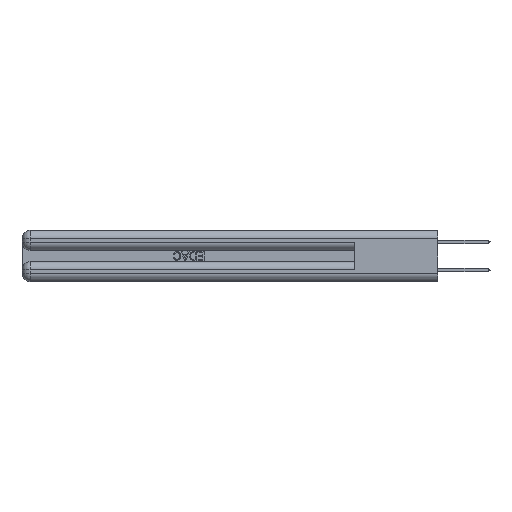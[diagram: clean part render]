
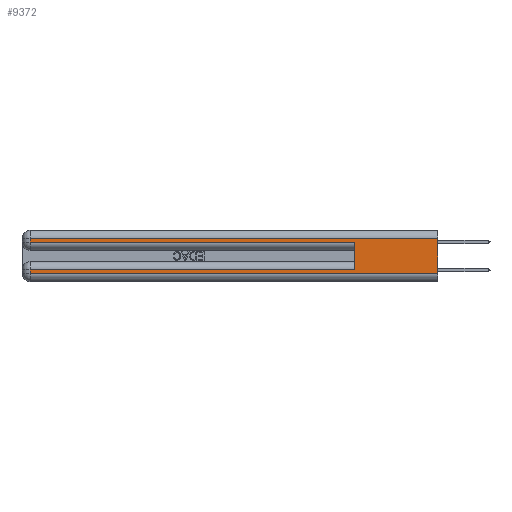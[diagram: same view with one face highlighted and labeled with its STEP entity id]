
A CAD part, left-side view. The second image highlights one B-rep face of the part: STEP entity #9372.
In plain terms, the highlighted planar face has unit normal (-1, 0, 0).
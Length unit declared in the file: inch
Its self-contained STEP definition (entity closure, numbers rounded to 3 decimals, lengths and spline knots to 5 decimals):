
#1352 = ORIENTED_EDGE ( 'NONE', *, *, #23393, .F. ) ;
#1395 = CARTESIAN_POINT ( 'NONE',  ( 0., 0., 0.06 ) ) ;
#1538 = AXIS2_PLACEMENT_3D ( 'NONE', #1649, #22900, #4738 ) ;
#1649 = CARTESIAN_POINT ( 'NONE',  ( 0., 0., 0.37 ) ) ;
#1921 = CARTESIAN_POINT ( 'NONE',  ( 0., 2.94, 0.37 ) ) ;
#2109 = CARTESIAN_POINT ( 'NONE',  ( 0., 2.94, 0.285 ) ) ;
#2770 = EDGE_CURVE ( 'NONE', #29899, #12724, #16586, .T. ) ;
#2954 = EDGE_CURVE ( 'NONE', #16357, #20465, #37391, .T. ) ;
#4738 = DIRECTION ( 'NONE',  ( 0., 0., -1. ) ) ;
#5775 = EDGE_CURVE ( 'NONE', #25235, #28966, #29657, .T. ) ;
#5843 = LINE ( 'NONE', #32188, #36691 ) ;
#5880 = CARTESIAN_POINT ( 'NONE',  ( 0., 0., 0.31 ) ) ;
#6415 = ORIENTED_EDGE ( 'NONE', *, *, #24428, .F. ) ;
#7683 = EDGE_CURVE ( 'NONE', #28966, #15906, #28596, .T. ) ;
#7878 = CARTESIAN_POINT ( 'NONE',  ( 0., 0., 0.31 ) ) ;
#8790 = LINE ( 'NONE', #28663, #14994 ) ;
#9093 = DIRECTION ( 'NONE',  ( 0., 0., -1. ) ) ;
#9372 = ADVANCED_FACE ( 'NONE', ( #11109 ), #31648, .F. ) ;
#10496 = EDGE_CURVE ( 'NONE', #15906, #24957, #5843, .T. ) ;
#11109 = FACE_OUTER_BOUND ( 'NONE', #13323, .T. ) ;
#12724 = VERTEX_POINT ( 'NONE', #25999 ) ;
#13323 = EDGE_LOOP ( 'NONE', ( #1352, #27396, #30391, #27155, #6415, #21587, #18764, #22016 ) ) ;
#14994 = VECTOR ( 'NONE', #31612, 39.37008 ) ;
#15906 = VERTEX_POINT ( 'NONE', #2109 ) ;
#16357 = VERTEX_POINT ( 'NONE', #36798 ) ;
#16586 = LINE ( 'NONE', #1395, #31421 ) ;
#17430 = DIRECTION ( 'NONE',  ( 0., -1., 0. ) ) ;
#18209 = DIRECTION ( 'NONE',  ( 0., 1., 0. ) ) ;
#18764 = ORIENTED_EDGE ( 'NONE', *, *, #33256, .T. ) ;
#19622 = DIRECTION ( 'NONE',  ( 0., -1., 0. ) ) ;
#19754 = VECTOR ( 'NONE', #23133, 39.37008 ) ;
#20465 = VERTEX_POINT ( 'NONE', #37831 ) ;
#21587 = ORIENTED_EDGE ( 'NONE', *, *, #2954, .T. ) ;
#22016 = ORIENTED_EDGE ( 'NONE', *, *, #2770, .T. ) ;
#22480 = DIRECTION ( 'NONE',  ( 0., 0., 1. ) ) ;
#22595 = VECTOR ( 'NONE', #9093, 39.37008 ) ;
#22900 = DIRECTION ( 'NONE',  ( 1., 0., 0. ) ) ;
#23133 = DIRECTION ( 'NONE',  ( 0., 0., -1. ) ) ;
#23393 = EDGE_CURVE ( 'NONE', #25235, #12724, #38237, .T. ) ;
#24127 = CARTESIAN_POINT ( 'NONE',  ( 0., 0., 0.37 ) ) ;
#24428 = EDGE_CURVE ( 'NONE', #16357, #24957, #32622, .T. ) ;
#24835 = VECTOR ( 'NONE', #22480, 39.37008 ) ;
#24957 = VERTEX_POINT ( 'NONE', #33507 ) ;
#25235 = VERTEX_POINT ( 'NONE', #7878 ) ;
#25999 = CARTESIAN_POINT ( 'NONE',  ( 0., 0., 0.06 ) ) ;
#26832 = VECTOR ( 'NONE', #18209, 39.37008 ) ;
#27064 = CARTESIAN_POINT ( 'NONE',  ( 0., 0., 0.085 ) ) ;
#27155 = ORIENTED_EDGE ( 'NONE', *, *, #10496, .T. ) ;
#27396 = ORIENTED_EDGE ( 'NONE', *, *, #5775, .T. ) ;
#28596 = LINE ( 'NONE', #1921, #19754 ) ;
#28663 = CARTESIAN_POINT ( 'NONE',  ( 0., 2.94, 0.37 ) ) ;
#28966 = VERTEX_POINT ( 'NONE', #38575 ) ;
#29657 = LINE ( 'NONE', #5880, #36529 ) ;
#29899 = VERTEX_POINT ( 'NONE', #31322 ) ;
#30391 = ORIENTED_EDGE ( 'NONE', *, *, #7683, .T. ) ;
#31240 = CARTESIAN_POINT ( 'NONE',  ( 0., 0.6, 0.145 ) ) ;
#31322 = CARTESIAN_POINT ( 'NONE',  ( 0., 2.94, 0.06 ) ) ;
#31421 = VECTOR ( 'NONE', #19622, 39.37008 ) ;
#31612 = DIRECTION ( 'NONE',  ( 0., 0., -1. ) ) ;
#31648 = PLANE ( 'NONE',  #1538 ) ;
#32188 = CARTESIAN_POINT ( 'NONE',  ( 0., 0., 0.285 ) ) ;
#32622 = LINE ( 'NONE', #31240, #24835 ) ;
#32855 = DIRECTION ( 'NONE',  ( 0., 1., 0. ) ) ;
#33256 = EDGE_CURVE ( 'NONE', #20465, #29899, #8790, .T. ) ;
#33507 = CARTESIAN_POINT ( 'NONE',  ( 0., 0.6, 0.285 ) ) ;
#36529 = VECTOR ( 'NONE', #32855, 39.37008 ) ;
#36691 = VECTOR ( 'NONE', #17430, 39.37008 ) ;
#36798 = CARTESIAN_POINT ( 'NONE',  ( 0., 0.6, 0.085 ) ) ;
#37391 = LINE ( 'NONE', #27064, #26832 ) ;
#37831 = CARTESIAN_POINT ( 'NONE',  ( 0., 2.94, 0.085 ) ) ;
#38237 = LINE ( 'NONE', #24127, #22595 ) ;
#38575 = CARTESIAN_POINT ( 'NONE',  ( 0., 2.94, 0.31 ) ) ;
